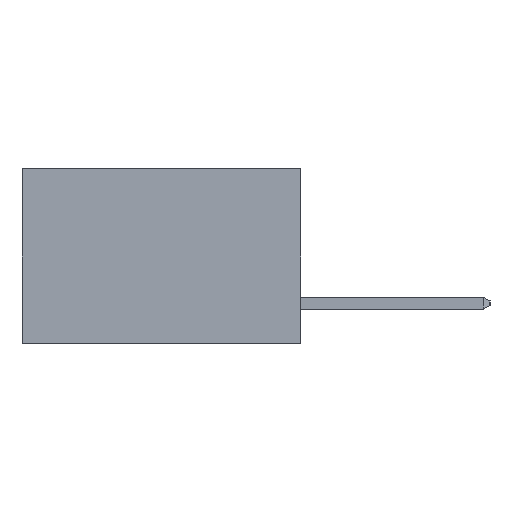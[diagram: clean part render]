
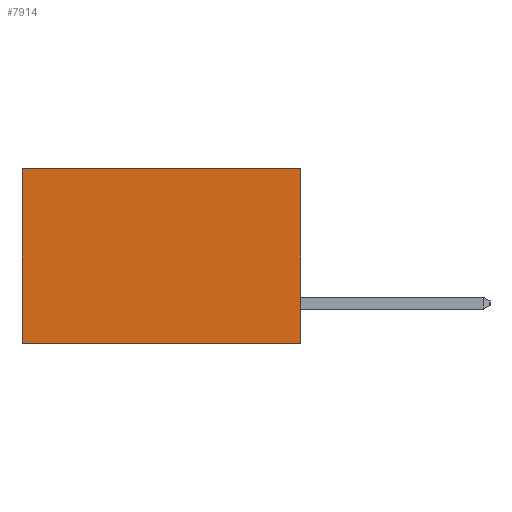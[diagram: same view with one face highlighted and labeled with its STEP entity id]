
A CAD part, left-side view. The second image highlights one B-rep face of the part: STEP entity #7914.
In plain terms, the highlighted planar face has unit normal (-1, 0, 0).
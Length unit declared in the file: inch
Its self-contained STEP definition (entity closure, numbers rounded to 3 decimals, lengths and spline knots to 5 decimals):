
#923 = ORIENTED_EDGE ( 'NONE', *, *, #10060, .T. ) ;
#1882 = DIRECTION ( 'NONE',  ( 0., 1., 0. ) ) ;
#2328 = DIRECTION ( 'NONE',  ( 0., 0., -1. ) ) ;
#2479 = CARTESIAN_POINT ( 'NONE',  ( 0.277, 0., -0.37 ) ) ;
#3173 = AXIS2_PLACEMENT_3D ( 'NONE', #2479, #18077, #7868 ) ;
#3224 = VECTOR ( 'NONE', #2328, 39.37008 ) ;
#3244 = CARTESIAN_POINT ( 'NONE',  ( 0.277, 0., -0.37 ) ) ;
#3931 = VERTEX_POINT ( 'NONE', #15131 ) ;
#3974 = VECTOR ( 'NONE', #1882, 39.37008 ) ;
#4106 = EDGE_CURVE ( 'NONE', #3931, #6049, #9691, .T. ) ;
#4126 = FACE_OUTER_BOUND ( 'NONE', #15041, .T. ) ;
#4766 = VERTEX_POINT ( 'NONE', #3244 ) ;
#5281 = CARTESIAN_POINT ( 'NONE',  ( 0.277, 0., 0. ) ) ;
#6049 = VERTEX_POINT ( 'NONE', #7456 ) ;
#7456 = CARTESIAN_POINT ( 'NONE',  ( 0.277, 0.59, 0. ) ) ;
#7570 = LINE ( 'NONE', #16570, #8123 ) ;
#7775 = LINE ( 'NONE', #19757, #20726 ) ;
#7868 = DIRECTION ( 'NONE',  ( 0., 0., -1. ) ) ;
#7914 = ADVANCED_FACE ( 'NONE', ( #4126 ), #9542, .F. ) ;
#8123 = VECTOR ( 'NONE', #14869, 39.37008 ) ;
#9542 = PLANE ( 'NONE',  #3173 ) ;
#9691 = LINE ( 'NONE', #5281, #3974 ) ;
#10060 = EDGE_CURVE ( 'NONE', #6049, #18476, #7570, .T. ) ;
#14869 = DIRECTION ( 'NONE',  ( 0., 0., -1. ) ) ;
#15041 = EDGE_LOOP ( 'NONE', ( #923, #15960, #15558, #15092 ) ) ;
#15092 = ORIENTED_EDGE ( 'NONE', *, *, #4106, .T. ) ;
#15131 = CARTESIAN_POINT ( 'NONE',  ( 0.277, 0., 0. ) ) ;
#15558 = ORIENTED_EDGE ( 'NONE', *, *, #21869, .F. ) ;
#15960 = ORIENTED_EDGE ( 'NONE', *, *, #17448, .F. ) ;
#16570 = CARTESIAN_POINT ( 'NONE',  ( 0.277, 0.59, -0.37 ) ) ;
#17030 = LINE ( 'NONE', #21163, #3224 ) ;
#17448 = EDGE_CURVE ( 'NONE', #4766, #18476, #7775, .T. ) ;
#18077 = DIRECTION ( 'NONE',  ( 1., 0., 0. ) ) ;
#18476 = VERTEX_POINT ( 'NONE', #22102 ) ;
#19757 = CARTESIAN_POINT ( 'NONE',  ( 0.277, 0., -0.37 ) ) ;
#20726 = VECTOR ( 'NONE', #21427, 39.37008 ) ;
#21163 = CARTESIAN_POINT ( 'NONE',  ( 0.277, 0., -0.37 ) ) ;
#21427 = DIRECTION ( 'NONE',  ( 0., 1., 0. ) ) ;
#21869 = EDGE_CURVE ( 'NONE', #3931, #4766, #17030, .T. ) ;
#22102 = CARTESIAN_POINT ( 'NONE',  ( 0.277, 0.59, -0.37 ) ) ;
